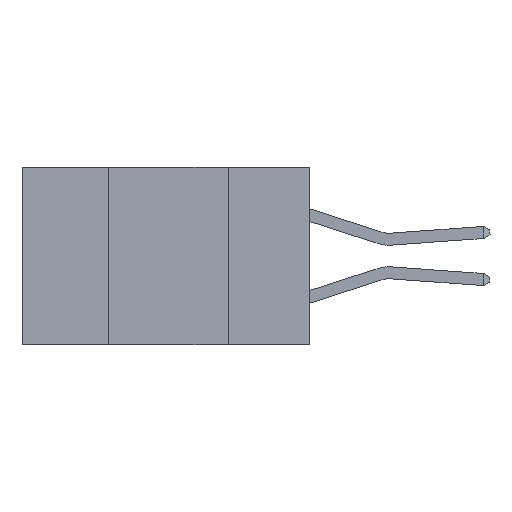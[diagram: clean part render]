
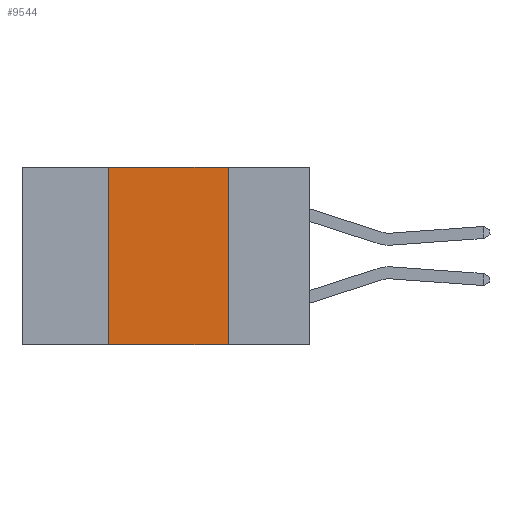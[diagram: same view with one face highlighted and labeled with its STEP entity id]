
A CAD part, left-side view. The second image highlights one B-rep face of the part: STEP entity #9544.
In plain terms, the highlighted planar face has unit normal (-1, 0, 0).
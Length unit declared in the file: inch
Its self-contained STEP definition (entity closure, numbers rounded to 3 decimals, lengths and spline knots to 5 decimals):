
#62 = DIRECTION ( 'NONE',  ( 0., 0., 1. ) ) ;
#746 = EDGE_CURVE ( 'NONE', #8516, #10133, #1212, .T. ) ;
#953 = EDGE_CURVE ( 'NONE', #11592, #5654, #13087, .T. ) ;
#1065 = LINE ( 'NONE', #11260, #8812 ) ;
#1212 = LINE ( 'NONE', #5527, #12593 ) ;
#1549 = EDGE_CURVE ( 'NONE', #5654, #10133, #14019, .T. ) ;
#1771 = ORIENTED_EDGE ( 'NONE', *, *, #746, .T. ) ;
#2016 = VECTOR ( 'NONE', #4138, 39.37008 ) ;
#2337 = EDGE_CURVE ( 'NONE', #8516, #11592, #1065, .T. ) ;
#2621 = DIRECTION ( 'NONE',  ( 0., -1., 0. ) ) ;
#2969 = CARTESIAN_POINT ( 'NONE',  ( 0., 0.6, 0. ) ) ;
#3059 = CARTESIAN_POINT ( 'NONE',  ( 0., 0.17, 0. ) ) ;
#4138 = DIRECTION ( 'NONE',  ( 0., 0., -1. ) ) ;
#5520 = DIRECTION ( 'NONE',  ( 1., 0., 0. ) ) ;
#5527 = CARTESIAN_POINT ( 'NONE',  ( 0., 0.6, -0.37 ) ) ;
#5654 = VERTEX_POINT ( 'NONE', #3059 ) ;
#5711 = CARTESIAN_POINT ( 'NONE',  ( 0., 0.42, -0.37 ) ) ;
#5811 = DIRECTION ( 'NONE',  ( 0., -1., 0. ) ) ;
#6167 = CARTESIAN_POINT ( 'NONE',  ( 0., 0.42, 0. ) ) ;
#6782 = AXIS2_PLACEMENT_3D ( 'NONE', #7241, #5520, #7221 ) ;
#6922 = PLANE ( 'NONE',  #6782 ) ;
#7221 = DIRECTION ( 'NONE',  ( 0., 0., -1. ) ) ;
#7222 = ORIENTED_EDGE ( 'NONE', *, *, #953, .F. ) ;
#7241 = CARTESIAN_POINT ( 'NONE',  ( 0., 0.6, 0. ) ) ;
#8516 = VERTEX_POINT ( 'NONE', #5711 ) ;
#8671 = CARTESIAN_POINT ( 'NONE',  ( 0., 0.17, -0.37 ) ) ;
#8812 = VECTOR ( 'NONE', #62, 39.37008 ) ;
#9544 = ADVANCED_FACE ( 'NONE', ( #14045 ), #6922, .F. ) ;
#9807 = VECTOR ( 'NONE', #5811, 39.37008 ) ;
#10133 = VERTEX_POINT ( 'NONE', #8671 ) ;
#10140 = ORIENTED_EDGE ( 'NONE', *, *, #1549, .F. ) ;
#10856 = EDGE_LOOP ( 'NONE', ( #10140, #7222, #13773, #1771 ) ) ;
#11260 = CARTESIAN_POINT ( 'NONE',  ( 0., 0.42, 0. ) ) ;
#11592 = VERTEX_POINT ( 'NONE', #6167 ) ;
#12508 = CARTESIAN_POINT ( 'NONE',  ( 0., 0.17, 0. ) ) ;
#12593 = VECTOR ( 'NONE', #2621, 39.37008 ) ;
#13087 = LINE ( 'NONE', #2969, #9807 ) ;
#13773 = ORIENTED_EDGE ( 'NONE', *, *, #2337, .F. ) ;
#14019 = LINE ( 'NONE', #12508, #2016 ) ;
#14045 = FACE_OUTER_BOUND ( 'NONE', #10856, .T. ) ;
